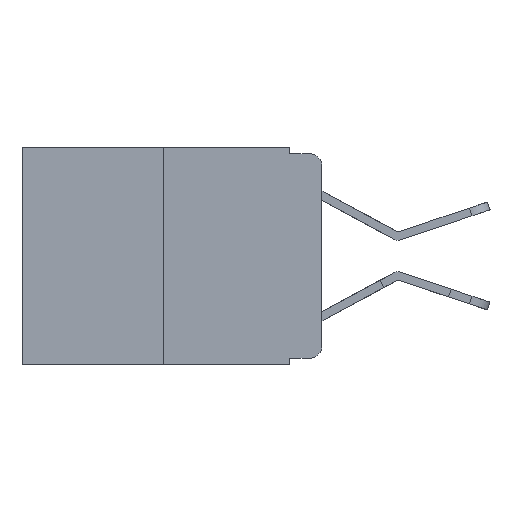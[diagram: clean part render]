
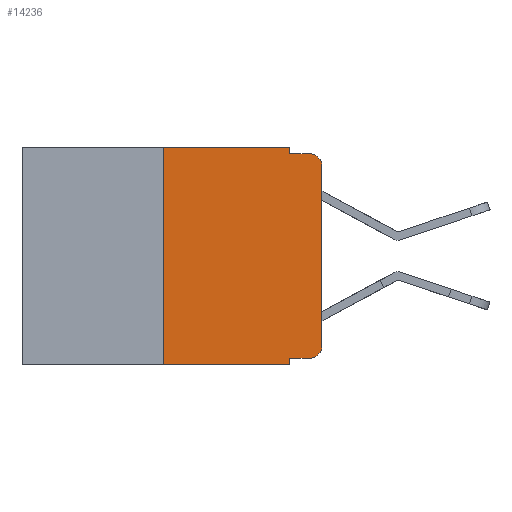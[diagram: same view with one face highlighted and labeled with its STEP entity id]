
A CAD part, left-side view. The second image highlights one B-rep face of the part: STEP entity #14236.
In plain terms, the highlighted planar face has unit normal (-1, 0, 0).
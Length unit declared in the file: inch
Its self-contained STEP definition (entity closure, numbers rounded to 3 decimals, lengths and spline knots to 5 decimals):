
#755 = VERTEX_POINT ( 'NONE', #25676 ) ;
#1404 = CARTESIAN_POINT ( 'NONE',  ( 0., 0.051, -0.333 ) ) ;
#1743 = VERTEX_POINT ( 'NONE', #18191 ) ;
#1760 = VECTOR ( 'NONE', #6351, 39.37008 ) ;
#1838 = VECTOR ( 'NONE', #10417, 39.37008 ) ;
#2074 = VECTOR ( 'NONE', #6715, 39.37008 ) ;
#2575 = EDGE_CURVE ( 'NONE', #14587, #2731, #4560, .T. ) ;
#2731 = VERTEX_POINT ( 'NONE', #14052 ) ;
#2912 = FACE_OUTER_BOUND ( 'NONE', #4600, .T. ) ;
#3008 = VERTEX_POINT ( 'NONE', #17372 ) ;
#3895 = VECTOR ( 'NONE', #13694, 39.37008 ) ;
#3984 = EDGE_CURVE ( 'NONE', #11436, #1743, #9109, .T. ) ;
#4013 = ORIENTED_EDGE ( 'NONE', *, *, #21745, .T. ) ;
#4185 = CARTESIAN_POINT ( 'NONE',  ( 0., 0.25, 0. ) ) ;
#4268 = ORIENTED_EDGE ( 'NONE', *, *, #15093, .T. ) ;
#4560 = LINE ( 'NONE', #17848, #3895 ) ;
#4600 = EDGE_LOOP ( 'NONE', ( #4013, #4268, #5979, #6918, #7496, #8483, #8659, #8980, #9604, #10661 ) ) ;
#5933 = CARTESIAN_POINT ( 'NONE',  ( 0., 0., -0.313 ) ) ;
#5979 = ORIENTED_EDGE ( 'NONE', *, *, #6821, .F. ) ;
#6351 = DIRECTION ( 'NONE',  ( 0., -1., 0. ) ) ;
#6715 = DIRECTION ( 'NONE',  ( 0., 0., 1. ) ) ;
#6821 = EDGE_CURVE ( 'NONE', #1743, #755, #22866, .T. ) ;
#6918 = ORIENTED_EDGE ( 'NONE', *, *, #3984, .F. ) ;
#7238 = EDGE_CURVE ( 'NONE', #23020, #2731, #17552, .T. ) ;
#7496 = ORIENTED_EDGE ( 'NONE', *, *, #16055, .F. ) ;
#7642 = LINE ( 'NONE', #10804, #17837 ) ;
#7663 = CARTESIAN_POINT ( 'NONE',  ( 0., 0.473, -0.343 ) ) ;
#7668 = LINE ( 'NONE', #18900, #2074 ) ;
#8444 = VECTOR ( 'NONE', #25410, 39.37008 ) ;
#8483 = ORIENTED_EDGE ( 'NONE', *, *, #26134, .F. ) ;
#8584 = DIRECTION ( 'NONE',  ( -1., 0., 0. ) ) ;
#8659 = ORIENTED_EDGE ( 'NONE', *, *, #7238, .T. ) ;
#8980 = ORIENTED_EDGE ( 'NONE', *, *, #2575, .F. ) ;
#9093 = CIRCLE ( 'NONE', #13760, 0.02 ) ;
#9109 = LINE ( 'NONE', #23430, #8444 ) ;
#9604 = ORIENTED_EDGE ( 'NONE', *, *, #22233, .T. ) ;
#10417 = DIRECTION ( 'NONE',  ( 0., -1., 0. ) ) ;
#10661 = ORIENTED_EDGE ( 'NONE', *, *, #23568, .T. ) ;
#10804 = CARTESIAN_POINT ( 'NONE',  ( 0., 0.051, -0.333 ) ) ;
#10835 = DIRECTION ( 'NONE',  ( 0., 0., -1. ) ) ;
#11288 = DIRECTION ( 'NONE',  ( 0., 0., 1. ) ) ;
#11436 = VERTEX_POINT ( 'NONE', #13362 ) ;
#11623 = DIRECTION ( 'NONE',  ( -1., 0., 0. ) ) ;
#11757 = AXIS2_PLACEMENT_3D ( 'NONE', #20677, #8584, #22701 ) ;
#12501 = CARTESIAN_POINT ( 'NONE',  ( 0., 0.473, 0. ) ) ;
#12841 = VECTOR ( 'NONE', #11288, 39.37008 ) ;
#12845 = DIRECTION ( 'NONE',  ( 0., -1., 0. ) ) ;
#13356 = CARTESIAN_POINT ( 'NONE',  ( 0., 0.02, -0.333 ) ) ;
#13362 = CARTESIAN_POINT ( 'NONE',  ( 0., 0.051, 0. ) ) ;
#13694 = DIRECTION ( 'NONE',  ( 0., 0., -1. ) ) ;
#13760 = AXIS2_PLACEMENT_3D ( 'NONE', #23555, #11623, #25511 ) ;
#14052 = CARTESIAN_POINT ( 'NONE',  ( 0., 0.051, -0.343 ) ) ;
#14236 = ADVANCED_FACE ( 'NONE', ( #2912 ), #20801, .F. ) ;
#14587 = VERTEX_POINT ( 'NONE', #1404 ) ;
#14936 = CARTESIAN_POINT ( 'NONE',  ( 0., 0.25, -0.343 ) ) ;
#15093 = EDGE_CURVE ( 'NONE', #3008, #755, #9093, .T. ) ;
#16055 = EDGE_CURVE ( 'NONE', #17639, #11436, #18269, .T. ) ;
#17372 = CARTESIAN_POINT ( 'NONE',  ( 0., 0., -0.03 ) ) ;
#17552 = LINE ( 'NONE', #7663, #22218 ) ;
#17639 = VERTEX_POINT ( 'NONE', #4185 ) ;
#17813 = DIRECTION ( 'NONE',  ( 0., -1., 0. ) ) ;
#17837 = VECTOR ( 'NONE', #12845, 39.37008 ) ;
#17848 = CARTESIAN_POINT ( 'NONE',  ( 0., 0.051, 0. ) ) ;
#17899 = CIRCLE ( 'NONE', #11757, 0.02 ) ;
#17937 = AXIS2_PLACEMENT_3D ( 'NONE', #18822, #22814, #10835 ) ;
#18191 = CARTESIAN_POINT ( 'NONE',  ( 0., 0.051, -0.01 ) ) ;
#18269 = LINE ( 'NONE', #12501, #1838 ) ;
#18537 = CARTESIAN_POINT ( 'NONE',  ( 0., 0.051, -0.01 ) ) ;
#18789 = LINE ( 'NONE', #25216, #12841 ) ;
#18822 = CARTESIAN_POINT ( 'NONE',  ( 0., 0.473, 0. ) ) ;
#18900 = CARTESIAN_POINT ( 'NONE',  ( 0., 0., 0. ) ) ;
#20677 = CARTESIAN_POINT ( 'NONE',  ( 0., 0.02, -0.313 ) ) ;
#20801 = PLANE ( 'NONE',  #17937 ) ;
#21518 = VERTEX_POINT ( 'NONE', #5933 ) ;
#21745 = EDGE_CURVE ( 'NONE', #21518, #3008, #7668, .T. ) ;
#22218 = VECTOR ( 'NONE', #17813, 39.37008 ) ;
#22233 = EDGE_CURVE ( 'NONE', #14587, #24324, #7642, .T. ) ;
#22701 = DIRECTION ( 'NONE',  ( 0., 0., -1. ) ) ;
#22814 = DIRECTION ( 'NONE',  ( 1., 0., 0. ) ) ;
#22866 = LINE ( 'NONE', #18537, #1760 ) ;
#23020 = VERTEX_POINT ( 'NONE', #14936 ) ;
#23430 = CARTESIAN_POINT ( 'NONE',  ( 0., 0.051, 0. ) ) ;
#23555 = CARTESIAN_POINT ( 'NONE',  ( 0., 0.02, -0.03 ) ) ;
#23568 = EDGE_CURVE ( 'NONE', #24324, #21518, #17899, .T. ) ;
#24324 = VERTEX_POINT ( 'NONE', #13356 ) ;
#25216 = CARTESIAN_POINT ( 'NONE',  ( 0., 0.25, 0. ) ) ;
#25410 = DIRECTION ( 'NONE',  ( 0., 0., -1. ) ) ;
#25511 = DIRECTION ( 'NONE',  ( 0., 0., -1. ) ) ;
#25676 = CARTESIAN_POINT ( 'NONE',  ( 0., 0.02, -0.01 ) ) ;
#26134 = EDGE_CURVE ( 'NONE', #23020, #17639, #18789, .T. ) ;
